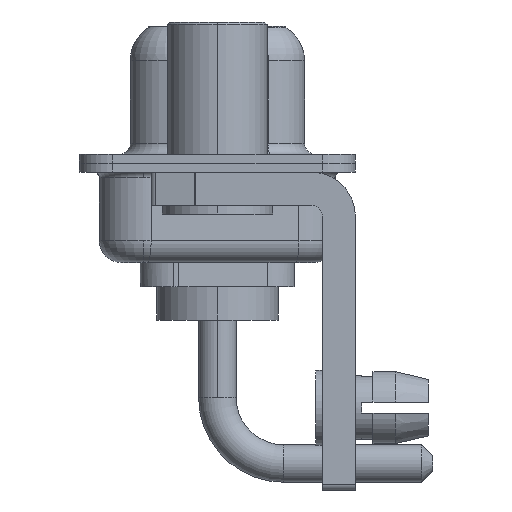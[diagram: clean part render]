
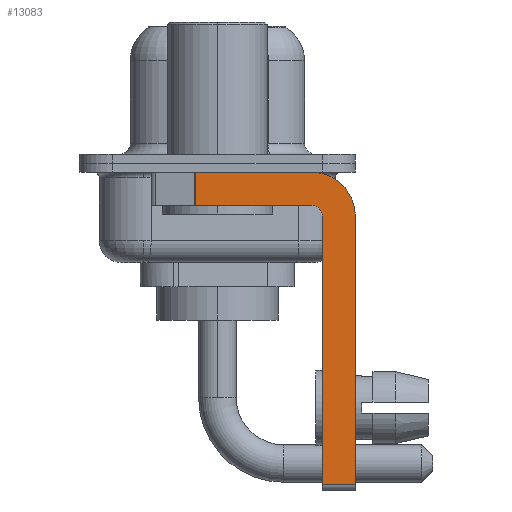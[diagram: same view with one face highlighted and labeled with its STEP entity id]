
A CAD part, left-side view. The second image highlights one B-rep face of the part: STEP entity #13083.
In plain terms, the highlighted planar face has unit normal (-1, 0, 0).
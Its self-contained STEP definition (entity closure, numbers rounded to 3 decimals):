
#17 = DIRECTION ( 'NONE',  ( 0., 0., -1. ) ) ;
#130 = VECTOR ( 'NONE', #7990, 1000. ) ;
#131 = CARTESIAN_POINT ( 'NONE',  ( -2.9, -6.25, -2.4 ) ) ;
#609 = EDGE_CURVE ( 'NONE', #14458, #7656, #5909, .T. ) ;
#624 = CARTESIAN_POINT ( 'NONE',  ( -2.9, -4.75, -2.4 ) ) ;
#642 = VERTEX_POINT ( 'NONE', #624 ) ;
#880 = CARTESIAN_POINT ( 'NONE',  ( -2.9, -6.25, -14.55 ) ) ;
#1168 = EDGE_CURVE ( 'NONE', #4633, #3177, #5597, .T. ) ;
#1182 = AXIS2_PLACEMENT_3D ( 'NONE', #10433, #11711, #17 ) ;
#1200 = EDGE_CURVE ( 'NONE', #642, #4633, #16605, .T. ) ;
#1236 = DIRECTION ( 'NONE',  ( 0., 0., -1. ) ) ;
#1241 = LINE ( 'NONE', #16773, #11307 ) ;
#1413 = ORIENTED_EDGE ( 'NONE', *, *, #609, .F. ) ;
#1655 = ORIENTED_EDGE ( 'NONE', *, *, #15181, .F. ) ;
#1852 = CARTESIAN_POINT ( 'NONE',  ( -2.9, -4.25, -1.9 ) ) ;
#1908 = VECTOR ( 'NONE', #5512, 1000. ) ;
#2436 = VERTEX_POINT ( 'NONE', #13728 ) ;
#2845 = FACE_OUTER_BOUND ( 'NONE', #8579, .T. ) ;
#3177 = VERTEX_POINT ( 'NONE', #13264 ) ;
#3878 = LINE ( 'NONE', #5258, #5554 ) ;
#4633 = VERTEX_POINT ( 'NONE', #8234 ) ;
#4875 = EDGE_CURVE ( 'NONE', #2436, #4976, #5145, .T. ) ;
#4976 = VERTEX_POINT ( 'NONE', #12037 ) ;
#5074 = DIRECTION ( 'NONE',  ( 1., 0., 0. ) ) ;
#5104 = ORIENTED_EDGE ( 'NONE', *, *, #14444, .T. ) ;
#5145 = LINE ( 'NONE', #11532, #11888 ) ;
#5258 = CARTESIAN_POINT ( 'NONE',  ( -2.9, 0.978, -1.9 ) ) ;
#5512 = DIRECTION ( 'NONE',  ( 0., 1., 0. ) ) ;
#5554 = VECTOR ( 'NONE', #1236, 1000. ) ;
#5597 = LINE ( 'NONE', #1852, #1908 ) ;
#5800 = CARTESIAN_POINT ( 'NONE',  ( -2.9, -4.75, -14.55 ) ) ;
#5909 = LINE ( 'NONE', #6070, #8708 ) ;
#6070 = CARTESIAN_POINT ( 'NONE',  ( -2.9, -6.25, -2.4 ) ) ;
#6255 = AXIS2_PLACEMENT_3D ( 'NONE', #14973, #8168, #9618 ) ;
#6495 = DIRECTION ( 'NONE',  ( 0., -1., 0. ) ) ;
#6516 = CARTESIAN_POINT ( 'NONE',  ( -2.9, -4.25, -2.4 ) ) ;
#6671 = AXIS2_PLACEMENT_3D ( 'NONE', #6516, #5074, #11718 ) ;
#7107 = ORIENTED_EDGE ( 'NONE', *, *, #1168, .F. ) ;
#7656 = VERTEX_POINT ( 'NONE', #880 ) ;
#7990 = DIRECTION ( 'NONE',  ( 0., 0., 1. ) ) ;
#8047 = PLANE ( 'NONE',  #1182 ) ;
#8168 = DIRECTION ( 'NONE',  ( -1., 0., 0. ) ) ;
#8234 = CARTESIAN_POINT ( 'NONE',  ( -2.9, -4.25, -1.9 ) ) ;
#8579 = EDGE_LOOP ( 'NONE', ( #13629, #5104, #7107, #12581, #1655, #12939, #1413, #13236 ) ) ;
#8708 = VECTOR ( 'NONE', #16318, 1000. ) ;
#8946 = CARTESIAN_POINT ( 'NONE',  ( -2.9, -4.75, -14.8 ) ) ;
#9618 = DIRECTION ( 'NONE',  ( 0., 0., 1. ) ) ;
#10433 = CARTESIAN_POINT ( 'NONE',  ( -2.9, -4.25, -2.4 ) ) ;
#11307 = VECTOR ( 'NONE', #11741, 1000. ) ;
#11532 = CARTESIAN_POINT ( 'NONE',  ( -2.9, 3., -0.4 ) ) ;
#11711 = DIRECTION ( 'NONE',  ( 1., 0., 0. ) ) ;
#11718 = DIRECTION ( 'NONE',  ( 0., 0., -1. ) ) ;
#11741 = DIRECTION ( 'NONE',  ( 0., -1., 0. ) ) ;
#11888 = VECTOR ( 'NONE', #6495, 1000. ) ;
#12037 = CARTESIAN_POINT ( 'NONE',  ( -2.9, -4.25, -0.4 ) ) ;
#12405 = CIRCLE ( 'NONE', #6671, 2. ) ;
#12581 = ORIENTED_EDGE ( 'NONE', *, *, #1200, .F. ) ;
#12939 = ORIENTED_EDGE ( 'NONE', *, *, #15081, .T. ) ;
#13083 = ADVANCED_FACE ( 'NONE', ( #2845 ), #8047, .F. ) ;
#13236 = ORIENTED_EDGE ( 'NONE', *, *, #15673, .F. ) ;
#13264 = CARTESIAN_POINT ( 'NONE',  ( -2.9, 0.978, -1.9 ) ) ;
#13629 = ORIENTED_EDGE ( 'NONE', *, *, #4875, .F. ) ;
#13679 = VERTEX_POINT ( 'NONE', #5800 ) ;
#13728 = CARTESIAN_POINT ( 'NONE',  ( -2.9, 0.978, -0.4 ) ) ;
#14444 = EDGE_CURVE ( 'NONE', #2436, #3177, #3878, .T. ) ;
#14458 = VERTEX_POINT ( 'NONE', #131 ) ;
#14460 = LINE ( 'NONE', #8946, #130 ) ;
#14973 = CARTESIAN_POINT ( 'NONE',  ( -2.9, -4.25, -2.4 ) ) ;
#15081 = EDGE_CURVE ( 'NONE', #13679, #7656, #1241, .T. ) ;
#15181 = EDGE_CURVE ( 'NONE', #13679, #642, #14460, .T. ) ;
#15673 = EDGE_CURVE ( 'NONE', #4976, #14458, #12405, .T. ) ;
#16318 = DIRECTION ( 'NONE',  ( 0., 0., -1. ) ) ;
#16605 = CIRCLE ( 'NONE', #6255, 0.5 ) ;
#16773 = CARTESIAN_POINT ( 'NONE',  ( -2.9, -4.25, -14.55 ) ) ;
